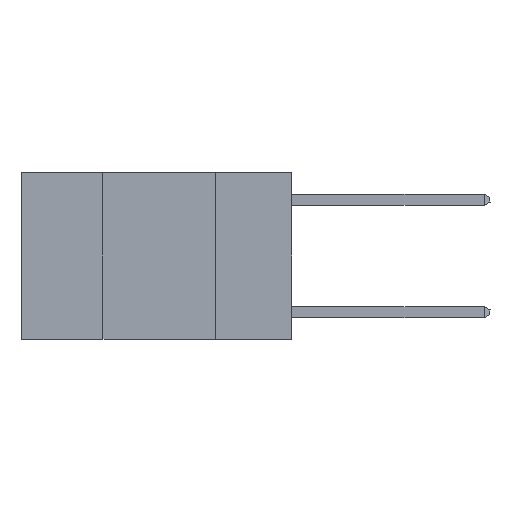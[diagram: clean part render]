
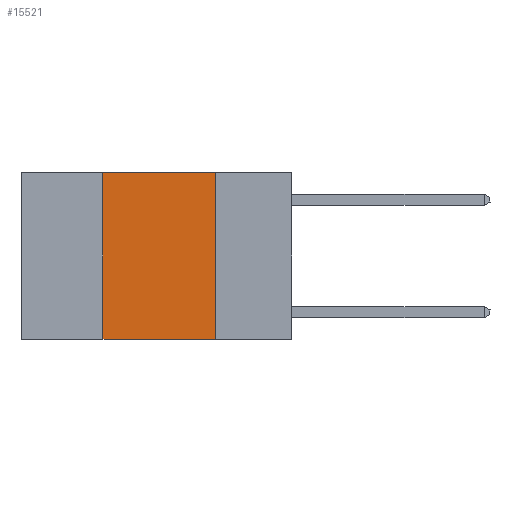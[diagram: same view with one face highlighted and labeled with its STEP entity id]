
A CAD part, left-side view. The second image highlights one B-rep face of the part: STEP entity #15521.
In plain terms, the highlighted planar face has unit normal (-1, 0, 0).
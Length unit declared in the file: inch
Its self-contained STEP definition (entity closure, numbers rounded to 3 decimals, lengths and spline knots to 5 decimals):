
#1274 = FACE_OUTER_BOUND ( 'NONE', #3647, .T. ) ;
#1559 = LINE ( 'NONE', #15200, #26993 ) ;
#1983 = VECTOR ( 'NONE', #13754, 39.37008 ) ;
#2255 = DIRECTION ( 'NONE',  ( 0., 0., 1. ) ) ;
#2735 = VECTOR ( 'NONE', #2255, 39.37008 ) ;
#3647 = EDGE_LOOP ( 'NONE', ( #25199, #7298, #11800, #16346 ) ) ;
#4120 = DIRECTION ( 'NONE',  ( 0., 0., -1. ) ) ;
#6759 = VERTEX_POINT ( 'NONE', #21170 ) ;
#7298 = ORIENTED_EDGE ( 'NONE', *, *, #29372, .F. ) ;
#7373 = EDGE_CURVE ( 'NONE', #8715, #6759, #25294, .T. ) ;
#7451 = VERTEX_POINT ( 'NONE', #14237 ) ;
#7632 = AXIS2_PLACEMENT_3D ( 'NONE', #19535, #12805, #26561 ) ;
#8715 = VERTEX_POINT ( 'NONE', #25300 ) ;
#9936 = CARTESIAN_POINT ( 'NONE',  ( 0., 0.6, -0.37 ) ) ;
#10416 = PLANE ( 'NONE',  #7632 ) ;
#11243 = CARTESIAN_POINT ( 'NONE',  ( 0., 0.17, -0.37 ) ) ;
#11800 = ORIENTED_EDGE ( 'NONE', *, *, #7373, .F. ) ;
#11878 = DIRECTION ( 'NONE',  ( 0., -1., 0. ) ) ;
#12805 = DIRECTION ( 'NONE',  ( 1., 0., 0. ) ) ;
#13510 = EDGE_CURVE ( 'NONE', #8715, #28919, #14268, .T. ) ;
#13754 = DIRECTION ( 'NONE',  ( 0., -1., 0. ) ) ;
#14199 = EDGE_CURVE ( 'NONE', #7451, #28919, #1559, .T. ) ;
#14237 = CARTESIAN_POINT ( 'NONE',  ( 0., 0.17, 0. ) ) ;
#14268 = LINE ( 'NONE', #9936, #16728 ) ;
#15200 = CARTESIAN_POINT ( 'NONE',  ( 0., 0.17, 0. ) ) ;
#15521 = ADVANCED_FACE ( 'NONE', ( #1274 ), #10416, .F. ) ;
#16346 = ORIENTED_EDGE ( 'NONE', *, *, #13510, .T. ) ;
#16728 = VECTOR ( 'NONE', #11878, 39.37008 ) ;
#19535 = CARTESIAN_POINT ( 'NONE',  ( 0., 0.6, 0. ) ) ;
#20767 = LINE ( 'NONE', #24816, #1983 ) ;
#21170 = CARTESIAN_POINT ( 'NONE',  ( 0., 0.42, 0. ) ) ;
#22752 = CARTESIAN_POINT ( 'NONE',  ( 0., 0.42, 0. ) ) ;
#24816 = CARTESIAN_POINT ( 'NONE',  ( 0., 0.6, 0. ) ) ;
#25199 = ORIENTED_EDGE ( 'NONE', *, *, #14199, .F. ) ;
#25294 = LINE ( 'NONE', #22752, #2735 ) ;
#25300 = CARTESIAN_POINT ( 'NONE',  ( 0., 0.42, -0.37 ) ) ;
#26561 = DIRECTION ( 'NONE',  ( 0., 0., -1. ) ) ;
#26993 = VECTOR ( 'NONE', #4120, 39.37008 ) ;
#28919 = VERTEX_POINT ( 'NONE', #11243 ) ;
#29372 = EDGE_CURVE ( 'NONE', #6759, #7451, #20767, .T. ) ;
